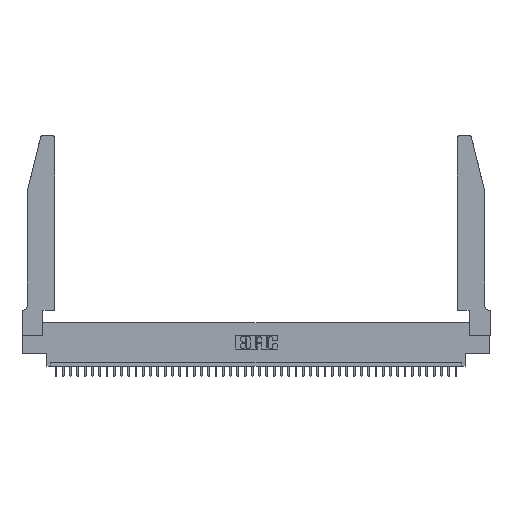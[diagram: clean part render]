
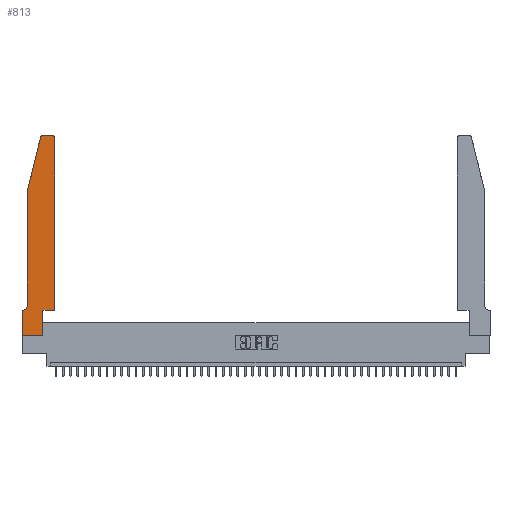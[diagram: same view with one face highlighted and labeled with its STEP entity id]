
A CAD part, top view. The second image highlights one B-rep face of the part: STEP entity #813.
In plain terms, the highlighted planar face has unit normal (0, 0, 1).
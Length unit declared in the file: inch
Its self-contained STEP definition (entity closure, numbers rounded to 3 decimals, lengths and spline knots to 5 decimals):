
#813 = ADVANCED_FACE ( 'NONE', ( #41805 ), #44838, .T. ) ;
#1561 = CARTESIAN_POINT ( 'NONE',  ( 0.25487, 2.72718, 0.37 ) ) ;
#1769 = DIRECTION ( 'NONE',  ( 0., 1., 0. ) ) ;
#2365 = ORIENTED_EDGE ( 'NONE', *, *, #23720, .T. ) ;
#3069 = CARTESIAN_POINT ( 'NONE',  ( 0., 0.35, 0.37 ) ) ;
#3457 = VERTEX_POINT ( 'NONE', #22465 ) ;
#3546 = LINE ( 'NONE', #6792, #39489 ) ;
#4047 = LINE ( 'NONE', #36881, #40097 ) ;
#4402 = CARTESIAN_POINT ( 'NONE',  ( 0., 0.35, 0.37 ) ) ;
#5296 = ORIENTED_EDGE ( 'NONE', *, *, #28530, .T. ) ;
#5565 = CARTESIAN_POINT ( 'NONE',  ( 0.2605, 2.75, 0.37 ) ) ;
#6599 = DIRECTION ( 'NONE',  ( 1., 0., 0. ) ) ;
#6629 = CARTESIAN_POINT ( 'NONE',  ( 0.4505, 0.35, 0.37 ) ) ;
#6792 = CARTESIAN_POINT ( 'NONE',  ( 0.4505, 0.35, 0.37 ) ) ;
#6886 = DIRECTION ( 'NONE',  ( 1., 0., 0. ) ) ;
#7335 = LINE ( 'NONE', #5565, #41216 ) ;
#7336 = CARTESIAN_POINT ( 'NONE',  ( 0.284, 2.75, 0.37 ) ) ;
#7373 = VERTEX_POINT ( 'NONE', #41680 ) ;
#7436 = DIRECTION ( 'NONE',  ( 0., -1., 0. ) ) ;
#8201 = EDGE_CURVE ( 'NONE', #43971, #30169, #33122, .T. ) ;
#10464 = AXIS2_PLACEMENT_3D ( 'NONE', #30274, #23338, #13160 ) ;
#11225 = CARTESIAN_POINT ( 'NONE',  ( 0.0755, 2., 0.37 ) ) ;
#11587 = EDGE_CURVE ( 'NONE', #43646, #20147, #15985, .T. ) ;
#12121 = DIRECTION ( 'NONE',  ( 0., 0., 1. ) ) ;
#12424 = ORIENTED_EDGE ( 'NONE', *, *, #8201, .T. ) ;
#12502 = DIRECTION ( 'NONE',  ( 0., 1., 0. ) ) ;
#13160 = DIRECTION ( 'NONE',  ( 1., 0., 0. ) ) ;
#14448 = ORIENTED_EDGE ( 'NONE', *, *, #42044, .T. ) ;
#15376 = CARTESIAN_POINT ( 'NONE',  ( 0.4505, 2.72, 0.37 ) ) ;
#15460 = LINE ( 'NONE', #26065, #37351 ) ;
#15831 = VERTEX_POINT ( 'NONE', #35021 ) ;
#15881 = CARTESIAN_POINT ( 'NONE',  ( 0., 0., 0.37 ) ) ;
#15985 = LINE ( 'NONE', #34627, #23044 ) ;
#17019 = VERTEX_POINT ( 'NONE', #33655 ) ;
#17547 = ORIENTED_EDGE ( 'NONE', *, *, #36978, .T. ) ;
#18836 = EDGE_CURVE ( 'NONE', #28025, #3457, #29505, .T. ) ;
#18921 = CARTESIAN_POINT ( 'NONE',  ( 0.284, 2.72, 0.37 ) ) ;
#19084 = VERTEX_POINT ( 'NONE', #4402 ) ;
#19677 = ORIENTED_EDGE ( 'NONE', *, *, #38360, .T. ) ;
#20147 = VERTEX_POINT ( 'NONE', #32494 ) ;
#20616 = LINE ( 'NONE', #43582, #30018 ) ;
#21274 = ORIENTED_EDGE ( 'NONE', *, *, #30351, .T. ) ;
#22223 = LINE ( 'NONE', #42790, #41963 ) ;
#22252 = CARTESIAN_POINT ( 'NONE',  ( 0.0055, 0.42, 0.37 ) ) ;
#22465 = CARTESIAN_POINT ( 'NONE',  ( 0.0755, 2., 0.37 ) ) ;
#22593 = EDGE_CURVE ( 'NONE', #33598, #28025, #43649, .T. ) ;
#22605 = CARTESIAN_POINT ( 'NONE',  ( 0.4505, 0.35, 0.37 ) ) ;
#22685 = CIRCLE ( 'NONE', #38556, 0.07 ) ;
#23044 = VECTOR ( 'NONE', #6886, 39.37008 ) ;
#23338 = DIRECTION ( 'NONE',  ( 0., 0., 1. ) ) ;
#23720 = EDGE_CURVE ( 'NONE', #19084, #43646, #20616, .T. ) ;
#25193 = DIRECTION ( 'NONE',  ( -1., 0., 0. ) ) ;
#26065 = CARTESIAN_POINT ( 'NONE',  ( 0.2865, 0.35, 0.37 ) ) ;
#26195 = EDGE_CURVE ( 'NONE', #17019, #33598, #7335, .T. ) ;
#27501 = DIRECTION ( 'NONE',  ( 0., 0., 1. ) ) ;
#27669 = ORIENTED_EDGE ( 'NONE', *, *, #26195, .T. ) ;
#28025 = VERTEX_POINT ( 'NONE', #1561 ) ;
#28530 = EDGE_CURVE ( 'NONE', #29514, #15831, #22685, .T. ) ;
#28930 = DIRECTION ( 'NONE',  ( 0., -1., 0. ) ) ;
#29505 = LINE ( 'NONE', #11225, #34434 ) ;
#29514 = VERTEX_POINT ( 'NONE', #39701 ) ;
#29981 = DIRECTION ( 'NONE',  ( -1., 0., 0. ) ) ;
#30018 = VECTOR ( 'NONE', #28930, 39.37008 ) ;
#30169 = VERTEX_POINT ( 'NONE', #15376 ) ;
#30274 = CARTESIAN_POINT ( 'NONE',  ( 0.4205, 2.72, 0.37 ) ) ;
#30351 = EDGE_CURVE ( 'NONE', #20147, #7373, #15460, .T. ) ;
#30846 = DIRECTION ( 'NONE',  ( -0.239, -0.971, 0. ) ) ;
#32494 = CARTESIAN_POINT ( 'NONE',  ( 0.2865, 0., 0.37 ) ) ;
#33122 = LINE ( 'NONE', #22605, #39089 ) ;
#33598 = VERTEX_POINT ( 'NONE', #7336 ) ;
#33655 = CARTESIAN_POINT ( 'NONE',  ( 0.4205, 2.75, 0.37 ) ) ;
#33664 = ORIENTED_EDGE ( 'NONE', *, *, #11587, .T. ) ;
#34069 = EDGE_CURVE ( 'NONE', #3457, #29514, #22223, .T. ) ;
#34237 = ORIENTED_EDGE ( 'NONE', *, *, #18836, .T. ) ;
#34434 = VECTOR ( 'NONE', #30846, 39.37008 ) ;
#34538 = CIRCLE ( 'NONE', #10464, 0.03 ) ;
#34627 = CARTESIAN_POINT ( 'NONE',  ( 0., 0., 0.37 ) ) ;
#35021 = CARTESIAN_POINT ( 'NONE',  ( 0.0055, 0.35, 0.37 ) ) ;
#36881 = CARTESIAN_POINT ( 'NONE',  ( 0.0755, 0.35, 0.37 ) ) ;
#36978 = EDGE_CURVE ( 'NONE', #15831, #19084, #4047, .T. ) ;
#37351 = VECTOR ( 'NONE', #12502, 39.37008 ) ;
#37612 = AXIS2_PLACEMENT_3D ( 'NONE', #18921, #12121, #42584 ) ;
#37813 = AXIS2_PLACEMENT_3D ( 'NONE', #3069, #27501, #6599 ) ;
#37996 = ORIENTED_EDGE ( 'NONE', *, *, #34069, .T. ) ;
#38169 = DIRECTION ( 'NONE',  ( 1., 0., 0. ) ) ;
#38360 = EDGE_CURVE ( 'NONE', #30169, #17019, #34538, .T. ) ;
#38556 = AXIS2_PLACEMENT_3D ( 'NONE', #22252, #42589, #25193 ) ;
#38784 = EDGE_LOOP ( 'NONE', ( #27669, #41037, #34237, #37996, #5296, #17547, #2365, #33664, #21274, #14448, #12424, #19677 ) ) ;
#39089 = VECTOR ( 'NONE', #1769, 39.37008 ) ;
#39489 = VECTOR ( 'NONE', #38169, 39.37008 ) ;
#39701 = CARTESIAN_POINT ( 'NONE',  ( 0.0755, 0.42, 0.37 ) ) ;
#40097 = VECTOR ( 'NONE', #40569, 39.37008 ) ;
#40569 = DIRECTION ( 'NONE',  ( -1., 0., 0. ) ) ;
#41037 = ORIENTED_EDGE ( 'NONE', *, *, #22593, .T. ) ;
#41216 = VECTOR ( 'NONE', #29981, 39.37008 ) ;
#41680 = CARTESIAN_POINT ( 'NONE',  ( 0.2865, 0.35, 0.37 ) ) ;
#41805 = FACE_OUTER_BOUND ( 'NONE', #38784, .T. ) ;
#41963 = VECTOR ( 'NONE', #7436, 39.37008 ) ;
#42044 = EDGE_CURVE ( 'NONE', #7373, #43971, #3546, .T. ) ;
#42584 = DIRECTION ( 'NONE',  ( 1., 0., 0. ) ) ;
#42589 = DIRECTION ( 'NONE',  ( 0., 0., -1. ) ) ;
#42790 = CARTESIAN_POINT ( 'NONE',  ( 0.0755, 2., 0.37 ) ) ;
#43582 = CARTESIAN_POINT ( 'NONE',  ( 0., 0., 0.37 ) ) ;
#43646 = VERTEX_POINT ( 'NONE', #15881 ) ;
#43649 = CIRCLE ( 'NONE', #37612, 0.03 ) ;
#43971 = VERTEX_POINT ( 'NONE', #6629 ) ;
#44838 = PLANE ( 'NONE',  #37813 ) ;
